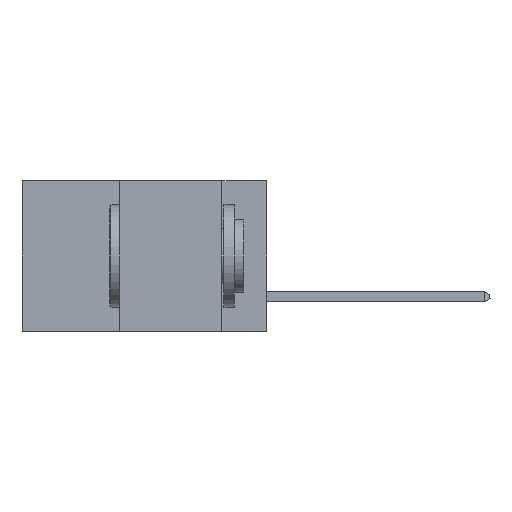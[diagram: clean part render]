
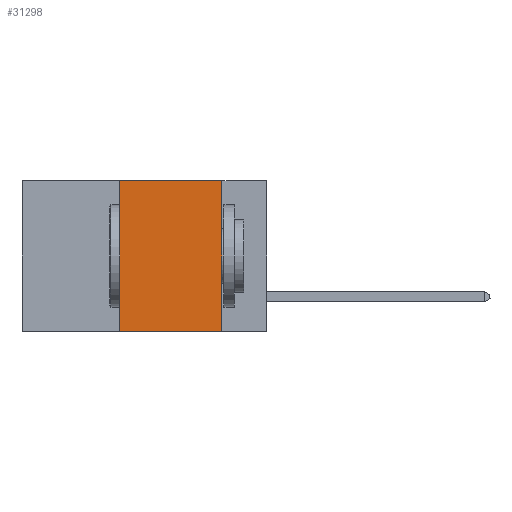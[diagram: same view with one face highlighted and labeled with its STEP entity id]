
A CAD part, left-side view. The second image highlights one B-rep face of the part: STEP entity #31298.
In plain terms, the highlighted planar face has unit normal (-1, 0, 0).
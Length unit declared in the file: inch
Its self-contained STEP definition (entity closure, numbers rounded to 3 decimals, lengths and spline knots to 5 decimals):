
#1707 = VECTOR ( 'NONE', #9262, 39.37008 ) ;
#2301 = VERTEX_POINT ( 'NONE', #31896 ) ;
#2799 = CARTESIAN_POINT ( 'NONE',  ( 0., 0.36, -0.37 ) ) ;
#2906 = VECTOR ( 'NONE', #5511, 39.37008 ) ;
#4481 = VECTOR ( 'NONE', #24538, 39.37008 ) ;
#5511 = DIRECTION ( 'NONE',  ( 0., -1., 0. ) ) ;
#7025 = ORIENTED_EDGE ( 'NONE', *, *, #28866, .F. ) ;
#7384 = CARTESIAN_POINT ( 'NONE',  ( 0., 0.11, 0. ) ) ;
#9262 = DIRECTION ( 'NONE',  ( 0., -1., 0. ) ) ;
#9902 = VERTEX_POINT ( 'NONE', #40447 ) ;
#10175 = EDGE_CURVE ( 'NONE', #9902, #2301, #25486, .T. ) ;
#10259 = CARTESIAN_POINT ( 'NONE',  ( 0., 0.6, 0. ) ) ;
#12247 = CARTESIAN_POINT ( 'NONE',  ( 0., 0.6, 0. ) ) ;
#16419 = LINE ( 'NONE', #12247, #1707 ) ;
#17232 = EDGE_CURVE ( 'NONE', #27567, #2301, #31344, .T. ) ;
#18223 = ORIENTED_EDGE ( 'NONE', *, *, #17232, .T. ) ;
#19568 = PLANE ( 'NONE',  #23813 ) ;
#19841 = DIRECTION ( 'NONE',  ( 0., 0., -1. ) ) ;
#21371 = CARTESIAN_POINT ( 'NONE',  ( 0., 0.36, 0. ) ) ;
#23810 = ORIENTED_EDGE ( 'NONE', *, *, #10175, .F. ) ;
#23813 = AXIS2_PLACEMENT_3D ( 'NONE', #10259, #38518, #19841 ) ;
#24333 = CARTESIAN_POINT ( 'NONE',  ( 0., 0.6, -0.37 ) ) ;
#24538 = DIRECTION ( 'NONE',  ( 0., 0., 1. ) ) ;
#24570 = CARTESIAN_POINT ( 'NONE',  ( 0., 0.36, 0. ) ) ;
#25486 = LINE ( 'NONE', #7384, #25953 ) ;
#25953 = VECTOR ( 'NONE', #26210, 39.37008 ) ;
#26210 = DIRECTION ( 'NONE',  ( 0., 0., -1. ) ) ;
#26563 = EDGE_LOOP ( 'NONE', ( #23810, #26687, #7025, #18223 ) ) ;
#26687 = ORIENTED_EDGE ( 'NONE', *, *, #40146, .F. ) ;
#27472 = FACE_OUTER_BOUND ( 'NONE', #26563, .T. ) ;
#27567 = VERTEX_POINT ( 'NONE', #2799 ) ;
#27730 = VERTEX_POINT ( 'NONE', #24570 ) ;
#28866 = EDGE_CURVE ( 'NONE', #27567, #27730, #34419, .T. ) ;
#31298 = ADVANCED_FACE ( 'NONE', ( #27472 ), #19568, .F. ) ;
#31344 = LINE ( 'NONE', #24333, #2906 ) ;
#31896 = CARTESIAN_POINT ( 'NONE',  ( 0., 0.11, -0.37 ) ) ;
#34419 = LINE ( 'NONE', #21371, #4481 ) ;
#38518 = DIRECTION ( 'NONE',  ( 1., 0., 0. ) ) ;
#40146 = EDGE_CURVE ( 'NONE', #27730, #9902, #16419, .T. ) ;
#40447 = CARTESIAN_POINT ( 'NONE',  ( 0., 0.11, 0. ) ) ;
